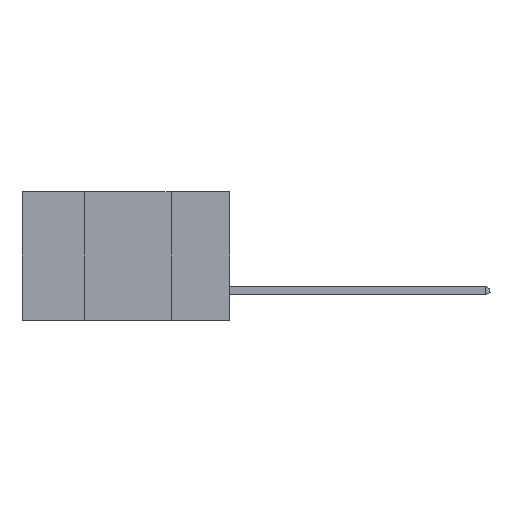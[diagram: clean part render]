
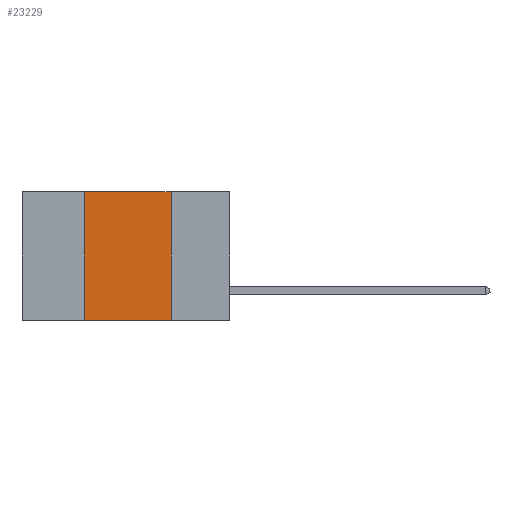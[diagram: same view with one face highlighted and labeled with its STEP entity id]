
A CAD part, left-side view. The second image highlights one B-rep face of the part: STEP entity #23229.
In plain terms, the highlighted planar face has unit normal (-1, 0, 0).
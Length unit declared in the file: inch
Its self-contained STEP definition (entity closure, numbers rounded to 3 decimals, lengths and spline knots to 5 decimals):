
#741 = LINE ( 'NONE', #20460, #9241 ) ;
#896 = FACE_OUTER_BOUND ( 'NONE', #18126, .T. ) ;
#972 = DIRECTION ( 'NONE',  ( 0., 0., -1. ) ) ;
#1483 = CARTESIAN_POINT ( 'NONE',  ( 0., 0.17, -0.37 ) ) ;
#2173 = CARTESIAN_POINT ( 'NONE',  ( 0., 0.6, -0.37 ) ) ;
#2440 = VERTEX_POINT ( 'NONE', #16728 ) ;
#4780 = DIRECTION ( 'NONE',  ( 0., -1., 0. ) ) ;
#5596 = VERTEX_POINT ( 'NONE', #1483 ) ;
#6317 = VECTOR ( 'NONE', #22717, 39.37008 ) ;
#7835 = CARTESIAN_POINT ( 'NONE',  ( 0., 0.6, 0. ) ) ;
#7976 = VECTOR ( 'NONE', #4780, 39.37008 ) ;
#7984 = DIRECTION ( 'NONE',  ( 0., 0., 1. ) ) ;
#9241 = VECTOR ( 'NONE', #7984, 39.37008 ) ;
#9332 = ORIENTED_EDGE ( 'NONE', *, *, #11884, .F. ) ;
#9905 = ORIENTED_EDGE ( 'NONE', *, *, #14420, .F. ) ;
#10990 = CARTESIAN_POINT ( 'NONE',  ( 0., 0.42, 0. ) ) ;
#11323 = LINE ( 'NONE', #13860, #21338 ) ;
#11884 = EDGE_CURVE ( 'NONE', #30709, #2440, #22530, .T. ) ;
#13422 = DIRECTION ( 'NONE',  ( 0., 0., -1. ) ) ;
#13860 = CARTESIAN_POINT ( 'NONE',  ( 0., 0.17, 0. ) ) ;
#14420 = EDGE_CURVE ( 'NONE', #21813, #30709, #741, .T. ) ;
#16728 = CARTESIAN_POINT ( 'NONE',  ( 0., 0.17, 0. ) ) ;
#18126 = EDGE_LOOP ( 'NONE', ( #30221, #9332, #9905, #25075 ) ) ;
#20460 = CARTESIAN_POINT ( 'NONE',  ( 0., 0.42, 0. ) ) ;
#20629 = CARTESIAN_POINT ( 'NONE',  ( 0., 0.6, 0. ) ) ;
#20926 = AXIS2_PLACEMENT_3D ( 'NONE', #20629, #23351, #972 ) ;
#21050 = PLANE ( 'NONE',  #20926 ) ;
#21338 = VECTOR ( 'NONE', #13422, 39.37008 ) ;
#21606 = EDGE_CURVE ( 'NONE', #2440, #5596, #11323, .T. ) ;
#21813 = VERTEX_POINT ( 'NONE', #31593 ) ;
#22530 = LINE ( 'NONE', #7835, #6317 ) ;
#22717 = DIRECTION ( 'NONE',  ( 0., -1., 0. ) ) ;
#23229 = ADVANCED_FACE ( 'NONE', ( #896 ), #21050, .F. ) ;
#23351 = DIRECTION ( 'NONE',  ( 1., 0., 0. ) ) ;
#25075 = ORIENTED_EDGE ( 'NONE', *, *, #27759, .T. ) ;
#27759 = EDGE_CURVE ( 'NONE', #21813, #5596, #28805, .T. ) ;
#28805 = LINE ( 'NONE', #2173, #7976 ) ;
#30221 = ORIENTED_EDGE ( 'NONE', *, *, #21606, .F. ) ;
#30709 = VERTEX_POINT ( 'NONE', #10990 ) ;
#31593 = CARTESIAN_POINT ( 'NONE',  ( 0., 0.42, -0.37 ) ) ;
